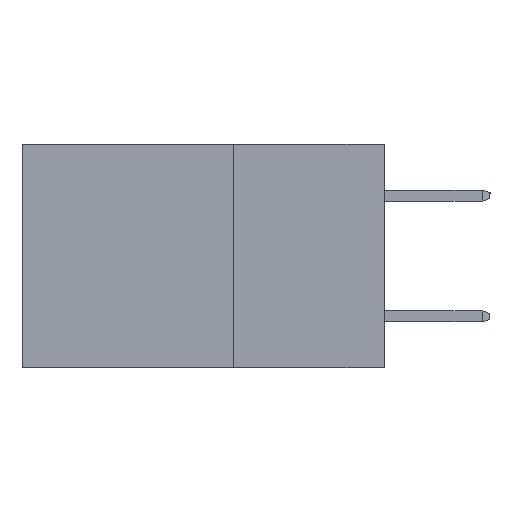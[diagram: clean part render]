
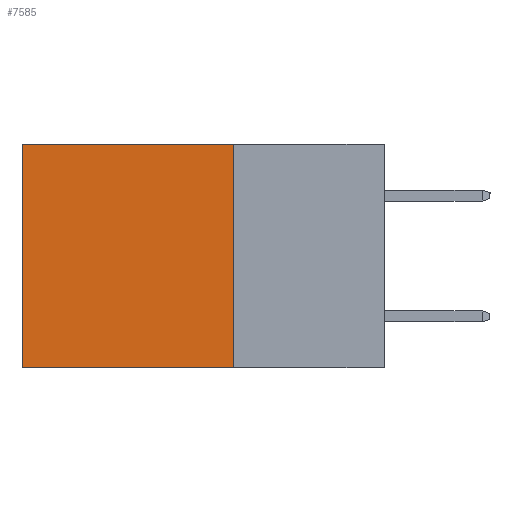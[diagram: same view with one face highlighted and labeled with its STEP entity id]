
A CAD part, left-side view. The second image highlights one B-rep face of the part: STEP entity #7585.
In plain terms, the highlighted planar face has unit normal (-1, 0, 0).
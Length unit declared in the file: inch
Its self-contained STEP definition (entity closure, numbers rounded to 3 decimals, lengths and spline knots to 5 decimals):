
#1057 = CARTESIAN_POINT ( 'NONE',  ( 0.2615, 0.25, -0.37 ) ) ;
#1084 = LINE ( 'NONE', #10120, #3809 ) ;
#1451 = CARTESIAN_POINT ( 'NONE',  ( 0.2615, 0.25, -0.37 ) ) ;
#2608 = FACE_OUTER_BOUND ( 'NONE', #3464, .T. ) ;
#2782 = EDGE_CURVE ( 'NONE', #3263, #4177, #4389, .T. ) ;
#3263 = VERTEX_POINT ( 'NONE', #6707 ) ;
#3464 = EDGE_LOOP ( 'NONE', ( #4317, #10105, #15207, #3575 ) ) ;
#3575 = ORIENTED_EDGE ( 'NONE', *, *, #16884, .T. ) ;
#3809 = VECTOR ( 'NONE', #9923, 39.37008 ) ;
#4177 = VERTEX_POINT ( 'NONE', #9700 ) ;
#4317 = ORIENTED_EDGE ( 'NONE', *, *, #13292, .T. ) ;
#4389 = LINE ( 'NONE', #1451, #11204 ) ;
#4720 = VERTEX_POINT ( 'NONE', #14163 ) ;
#5954 = DIRECTION ( 'NONE',  ( 0., 1., 0. ) ) ;
#6707 = CARTESIAN_POINT ( 'NONE',  ( 0.2615, 0.25, -0.37 ) ) ;
#6740 = LINE ( 'NONE', #12733, #19095 ) ;
#7585 = ADVANCED_FACE ( 'NONE', ( #2608 ), #9965, .F. ) ;
#8131 = VERTEX_POINT ( 'NONE', #10699 ) ;
#8589 = DIRECTION ( 'NONE',  ( 0., 0., -1. ) ) ;
#8727 = DIRECTION ( 'NONE',  ( 0., 0., -1. ) ) ;
#9700 = CARTESIAN_POINT ( 'NONE',  ( 0.2615, 0.6, -0.37 ) ) ;
#9893 = LINE ( 'NONE', #1057, #13824 ) ;
#9923 = DIRECTION ( 'NONE',  ( 0., 1., 0. ) ) ;
#9965 = PLANE ( 'NONE',  #10550 ) ;
#10105 = ORIENTED_EDGE ( 'NONE', *, *, #2782, .F. ) ;
#10120 = CARTESIAN_POINT ( 'NONE',  ( 0.2615, 0.25, 0. ) ) ;
#10550 = AXIS2_PLACEMENT_3D ( 'NONE', #15968, #12995, #8589 ) ;
#10699 = CARTESIAN_POINT ( 'NONE',  ( 0.2615, 0.25, 0. ) ) ;
#11204 = VECTOR ( 'NONE', #5954, 39.37008 ) ;
#12733 = CARTESIAN_POINT ( 'NONE',  ( 0.2615, 0.6, -0.37 ) ) ;
#12995 = DIRECTION ( 'NONE',  ( 1., 0., 0. ) ) ;
#13292 = EDGE_CURVE ( 'NONE', #4720, #4177, #6740, .T. ) ;
#13824 = VECTOR ( 'NONE', #8727, 39.37008 ) ;
#14163 = CARTESIAN_POINT ( 'NONE',  ( 0.2615, 0.6, 0. ) ) ;
#15207 = ORIENTED_EDGE ( 'NONE', *, *, #16013, .F. ) ;
#15968 = CARTESIAN_POINT ( 'NONE',  ( 0.2615, 0.25, -0.37 ) ) ;
#16013 = EDGE_CURVE ( 'NONE', #8131, #3263, #9893, .T. ) ;
#16884 = EDGE_CURVE ( 'NONE', #8131, #4720, #1084, .T. ) ;
#18745 = DIRECTION ( 'NONE',  ( 0., 0., -1. ) ) ;
#19095 = VECTOR ( 'NONE', #18745, 39.37008 ) ;
